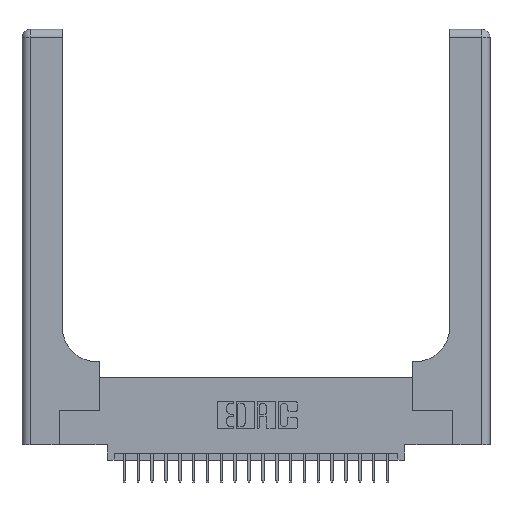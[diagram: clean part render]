
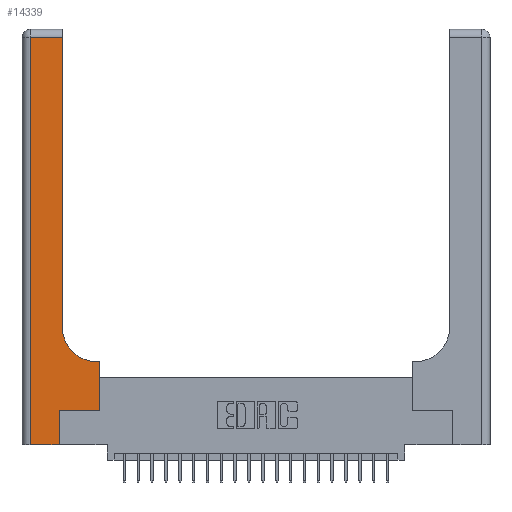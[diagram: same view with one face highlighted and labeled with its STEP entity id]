
A CAD part, top view. The second image highlights one B-rep face of the part: STEP entity #14339.
In plain terms, the highlighted planar face has unit normal (0, 0, 1).
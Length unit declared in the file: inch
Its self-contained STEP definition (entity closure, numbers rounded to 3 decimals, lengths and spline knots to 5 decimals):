
#834 = VECTOR ( 'NONE', #8924, 39.37008 ) ;
#1066 = LINE ( 'NONE', #19498, #8339 ) ;
#1485 = VERTEX_POINT ( 'NONE', #12914 ) ;
#1623 = CIRCLE ( 'NONE', #17470, 0.25 ) ;
#1652 = VERTEX_POINT ( 'NONE', #8757 ) ;
#1831 = VERTEX_POINT ( 'NONE', #6620 ) ;
#2025 = EDGE_CURVE ( 'NONE', #1652, #1831, #15643, .T. ) ;
#2322 = DIRECTION ( 'NONE',  ( -1., 0., 0. ) ) ;
#2554 = EDGE_CURVE ( 'NONE', #5101, #18100, #15618, .T. ) ;
#2576 = VERTEX_POINT ( 'NONE', #3321 ) ;
#2799 = DIRECTION ( 'NONE',  ( -1., 0., 0. ) ) ;
#3221 = EDGE_CURVE ( 'NONE', #18942, #1485, #21445, .T. ) ;
#3321 = CARTESIAN_POINT ( 'NONE',  ( 0.06, 2.94, 0.37 ) ) ;
#3582 = DIRECTION ( 'NONE',  ( 0., 1., 0. ) ) ;
#3917 = AXIS2_PLACEMENT_3D ( 'NONE', #12005, #8570, #2799 ) ;
#4482 = CARTESIAN_POINT ( 'NONE',  ( 0.269, 0., 0.37 ) ) ;
#5101 = VERTEX_POINT ( 'NONE', #6679 ) ;
#6018 = CARTESIAN_POINT ( 'NONE',  ( 0., 0., 0.37 ) ) ;
#6192 = EDGE_CURVE ( 'NONE', #1831, #2576, #9192, .T. ) ;
#6592 = FACE_OUTER_BOUND ( 'NONE', #19011, .T. ) ;
#6620 = CARTESIAN_POINT ( 'NONE',  ( 0.2915, 2.94, 0.37 ) ) ;
#6679 = CARTESIAN_POINT ( 'NONE',  ( 0.5585, 0.25, 0.37 ) ) ;
#7328 = LINE ( 'NONE', #14919, #10503 ) ;
#7728 = DIRECTION ( 'NONE',  ( 1., 0., 0. ) ) ;
#8287 = DIRECTION ( 'NONE',  ( 0., 1., 0. ) ) ;
#8323 = EDGE_CURVE ( 'NONE', #1485, #5101, #7328, .T. ) ;
#8339 = VECTOR ( 'NONE', #18949, 39.37008 ) ;
#8570 = DIRECTION ( 'NONE',  ( 0., 0., -1. ) ) ;
#8757 = CARTESIAN_POINT ( 'NONE',  ( 0.2915, 0.85, 0.37 ) ) ;
#8924 = DIRECTION ( 'NONE',  ( 0., 1., 0. ) ) ;
#9192 = LINE ( 'NONE', #12947, #12880 ) ;
#10421 = EDGE_CURVE ( 'NONE', #18100, #23149, #22034, .T. ) ;
#10503 = VECTOR ( 'NONE', #13116, 39.37008 ) ;
#10526 = VECTOR ( 'NONE', #16970, 39.37008 ) ;
#10864 = ORIENTED_EDGE ( 'NONE', *, *, #2025, .T. ) ;
#11181 = EDGE_CURVE ( 'NONE', #2576, #14824, #1066, .T. ) ;
#11562 = CARTESIAN_POINT ( 'NONE',  ( 0.5415, 0.85, 0.37 ) ) ;
#11817 = VECTOR ( 'NONE', #2322, 39.37008 ) ;
#12005 = CARTESIAN_POINT ( 'NONE',  ( 0., 3., 0.37 ) ) ;
#12458 = ORIENTED_EDGE ( 'NONE', *, *, #10421, .T. ) ;
#12880 = VECTOR ( 'NONE', #20377, 39.37008 ) ;
#12914 = CARTESIAN_POINT ( 'NONE',  ( 0.269, 0.25, 0.37 ) ) ;
#12947 = CARTESIAN_POINT ( 'NONE',  ( 0., 2.94, 0.37 ) ) ;
#13116 = DIRECTION ( 'NONE',  ( 1., 0., 0. ) ) ;
#13820 = CARTESIAN_POINT ( 'NONE',  ( 0.269, 0., 0.37 ) ) ;
#13959 = CARTESIAN_POINT ( 'NONE',  ( 0.5415, 0.6, 0.37 ) ) ;
#13994 = LINE ( 'NONE', #6018, #10526 ) ;
#14156 = ORIENTED_EDGE ( 'NONE', *, *, #2554, .T. ) ;
#14339 = ADVANCED_FACE ( 'NONE', ( #6592 ), #19654, .F. ) ;
#14824 = VERTEX_POINT ( 'NONE', #20281 ) ;
#14919 = CARTESIAN_POINT ( 'NONE',  ( 0.269, 0.25, 0.37 ) ) ;
#15475 = DIRECTION ( 'NONE',  ( 0., 0., -1. ) ) ;
#15618 = LINE ( 'NONE', #19846, #834 ) ;
#15643 = LINE ( 'NONE', #18262, #18856 ) ;
#16467 = VECTOR ( 'NONE', #8287, 39.37008 ) ;
#16970 = DIRECTION ( 'NONE',  ( 1., 0., 0. ) ) ;
#17470 = AXIS2_PLACEMENT_3D ( 'NONE', #11562, #15475, #7728 ) ;
#17632 = ORIENTED_EDGE ( 'NONE', *, *, #3221, .T. ) ;
#17855 = ORIENTED_EDGE ( 'NONE', *, *, #21752, .T. ) ;
#17945 = ORIENTED_EDGE ( 'NONE', *, *, #23464, .T. ) ;
#17979 = ORIENTED_EDGE ( 'NONE', *, *, #6192, .T. ) ;
#18100 = VERTEX_POINT ( 'NONE', #23980 ) ;
#18262 = CARTESIAN_POINT ( 'NONE',  ( 0.2915, 3., 0.37 ) ) ;
#18856 = VECTOR ( 'NONE', #3582, 39.37008 ) ;
#18942 = VERTEX_POINT ( 'NONE', #4482 ) ;
#18949 = DIRECTION ( 'NONE',  ( 0., -1., 0. ) ) ;
#19011 = EDGE_LOOP ( 'NONE', ( #10864, #17979, #20581, #17945, #17632, #23914, #14156, #12458, #17855 ) ) ;
#19136 = CARTESIAN_POINT ( 'NONE',  ( 0.2915, 0.6, 0.37 ) ) ;
#19498 = CARTESIAN_POINT ( 'NONE',  ( 0.06, 3., 0.37 ) ) ;
#19654 = PLANE ( 'NONE',  #3917 ) ;
#19846 = CARTESIAN_POINT ( 'NONE',  ( 0.5585, 0.25, 0.37 ) ) ;
#20281 = CARTESIAN_POINT ( 'NONE',  ( 0.06, 0., 0.37 ) ) ;
#20377 = DIRECTION ( 'NONE',  ( -1., 0., 0. ) ) ;
#20581 = ORIENTED_EDGE ( 'NONE', *, *, #11181, .T. ) ;
#21445 = LINE ( 'NONE', #13820, #16467 ) ;
#21752 = EDGE_CURVE ( 'NONE', #23149, #1652, #1623, .T. ) ;
#22034 = LINE ( 'NONE', #19136, #11817 ) ;
#23149 = VERTEX_POINT ( 'NONE', #13959 ) ;
#23464 = EDGE_CURVE ( 'NONE', #14824, #18942, #13994, .T. ) ;
#23914 = ORIENTED_EDGE ( 'NONE', *, *, #8323, .T. ) ;
#23980 = CARTESIAN_POINT ( 'NONE',  ( 0.5585, 0.6, 0.37 ) ) ;
